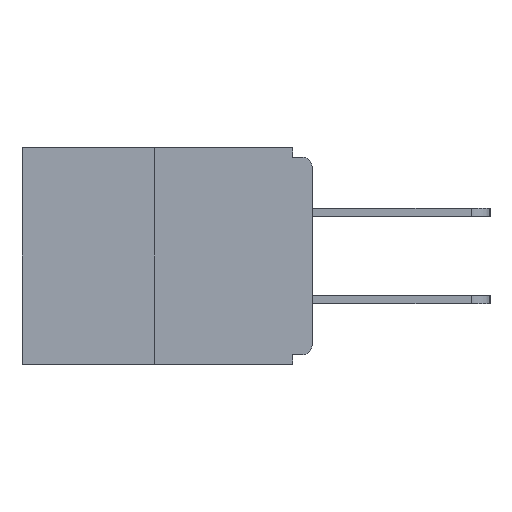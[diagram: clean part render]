
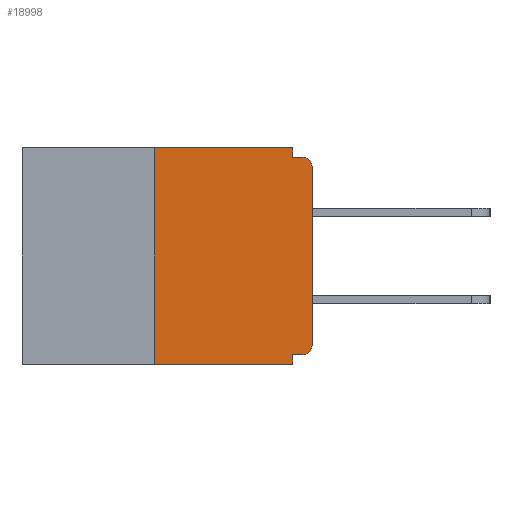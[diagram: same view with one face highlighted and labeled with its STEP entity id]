
A CAD part, left-side view. The second image highlights one B-rep face of the part: STEP entity #18998.
In plain terms, the highlighted planar face has unit normal (-1, 0, 0).
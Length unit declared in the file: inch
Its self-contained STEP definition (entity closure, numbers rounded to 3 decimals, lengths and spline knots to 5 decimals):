
#449 = DIRECTION ( 'NONE',  ( 0., 0., 1. ) ) ;
#732 = CARTESIAN_POINT ( 'NONE',  ( 0., 0.25, 0. ) ) ;
#2021 = CARTESIAN_POINT ( 'NONE',  ( 0., 0.25, -0.343 ) ) ;
#2976 = CARTESIAN_POINT ( 'NONE',  ( 0., 0., -0.328 ) ) ;
#3298 = LINE ( 'NONE', #7360, #22466 ) ;
#4478 = DIRECTION ( 'NONE',  ( 1., 0., 0. ) ) ;
#4510 = CARTESIAN_POINT ( 'NONE',  ( 0., 0.25, 0. ) ) ;
#4752 = VERTEX_POINT ( 'NONE', #18791 ) ;
#4906 = LINE ( 'NONE', #26805, #29667 ) ;
#4946 = EDGE_CURVE ( 'NONE', #25411, #9145, #12373, .T. ) ;
#5059 = EDGE_LOOP ( 'NONE', ( #11065, #24870, #18500, #27363, #10244, #5764, #27977, #21273, #30615, #14819 ) ) ;
#5166 = EDGE_CURVE ( 'NONE', #6661, #10984, #5220, .T. ) ;
#5220 = CIRCLE ( 'NONE', #25981, 0.015 ) ;
#5764 = ORIENTED_EDGE ( 'NONE', *, *, #5166, .T. ) ;
#6032 = FACE_OUTER_BOUND ( 'NONE', #5059, .T. ) ;
#6065 = DIRECTION ( 'NONE',  ( -1., 0., 0. ) ) ;
#6290 = CARTESIAN_POINT ( 'NONE',  ( 0., 0.031, 0. ) ) ;
#6461 = PLANE ( 'NONE',  #17625 ) ;
#6661 = VERTEX_POINT ( 'NONE', #27737 ) ;
#7360 = CARTESIAN_POINT ( 'NONE',  ( 0., 0., -0.015 ) ) ;
#7585 = VECTOR ( 'NONE', #449, 39.37008 ) ;
#9145 = VERTEX_POINT ( 'NONE', #24005 ) ;
#9698 = LINE ( 'NONE', #2976, #14955 ) ;
#10244 = ORIENTED_EDGE ( 'NONE', *, *, #13657, .F. ) ;
#10552 = CARTESIAN_POINT ( 'NONE',  ( 0., 0.46, -0.343 ) ) ;
#10764 = LINE ( 'NONE', #10552, #26503 ) ;
#10984 = VERTEX_POINT ( 'NONE', #27610 ) ;
#11065 = ORIENTED_EDGE ( 'NONE', *, *, #12440, .F. ) ;
#12373 = LINE ( 'NONE', #30499, #13145 ) ;
#12437 = DIRECTION ( 'NONE',  ( 0., -1., 0. ) ) ;
#12440 = EDGE_CURVE ( 'NONE', #20404, #25411, #4906, .T. ) ;
#12599 = CARTESIAN_POINT ( 'NONE',  ( 0., 0., -0.03 ) ) ;
#12611 = EDGE_CURVE ( 'NONE', #28470, #19201, #10764, .T. ) ;
#13145 = VECTOR ( 'NONE', #30386, 39.37008 ) ;
#13269 = CARTESIAN_POINT ( 'NONE',  ( 0., 0.031, -0.343 ) ) ;
#13657 = EDGE_CURVE ( 'NONE', #6661, #17230, #9698, .T. ) ;
#13726 = DIRECTION ( 'NONE',  ( 0., 0., -1. ) ) ;
#14003 = DIRECTION ( 'NONE',  ( 0., 0., -1. ) ) ;
#14268 = DIRECTION ( 'NONE',  ( 0., 0., 1. ) ) ;
#14388 = VECTOR ( 'NONE', #14268, 39.37008 ) ;
#14644 = CIRCLE ( 'NONE', #20902, 0.015 ) ;
#14819 = ORIENTED_EDGE ( 'NONE', *, *, #4946, .F. ) ;
#14955 = VECTOR ( 'NONE', #26798, 39.37008 ) ;
#15053 = DIRECTION ( 'NONE',  ( -1., 0., 0. ) ) ;
#15155 = CARTESIAN_POINT ( 'NONE',  ( 0., 0.015, -0.313 ) ) ;
#15611 = CARTESIAN_POINT ( 'NONE',  ( 0., 0.031, -0.328 ) ) ;
#16011 = DIRECTION ( 'NONE',  ( 0., 0., -1. ) ) ;
#16230 = LINE ( 'NONE', #19332, #7585 ) ;
#16352 = LINE ( 'NONE', #18699, #24613 ) ;
#17230 = VERTEX_POINT ( 'NONE', #15611 ) ;
#17379 = LINE ( 'NONE', #4510, #14388 ) ;
#17625 = AXIS2_PLACEMENT_3D ( 'NONE', #28490, #4478, #13726 ) ;
#17681 = EDGE_CURVE ( 'NONE', #10984, #21330, #16230, .T. ) ;
#18500 = ORIENTED_EDGE ( 'NONE', *, *, #12611, .T. ) ;
#18699 = CARTESIAN_POINT ( 'NONE',  ( 0., 0.031, -0.343 ) ) ;
#18791 = CARTESIAN_POINT ( 'NONE',  ( 0., 0.015, -0.015 ) ) ;
#18998 = ADVANCED_FACE ( 'NONE', ( #6032 ), #6461, .F. ) ;
#19201 = VERTEX_POINT ( 'NONE', #13269 ) ;
#19332 = CARTESIAN_POINT ( 'NONE',  ( 0., 0., 0. ) ) ;
#20404 = VERTEX_POINT ( 'NONE', #732 ) ;
#20902 = AXIS2_PLACEMENT_3D ( 'NONE', #30072, #6065, #16011 ) ;
#20904 = EDGE_CURVE ( 'NONE', #21330, #4752, #14644, .T. ) ;
#21273 = ORIENTED_EDGE ( 'NONE', *, *, #20904, .T. ) ;
#21330 = VERTEX_POINT ( 'NONE', #12599 ) ;
#22112 = EDGE_CURVE ( 'NONE', #9145, #4752, #3298, .T. ) ;
#22466 = VECTOR ( 'NONE', #24174, 39.37008 ) ;
#24005 = CARTESIAN_POINT ( 'NONE',  ( 0., 0.031, -0.015 ) ) ;
#24174 = DIRECTION ( 'NONE',  ( 0., -1., 0. ) ) ;
#24613 = VECTOR ( 'NONE', #14003, 39.37008 ) ;
#24870 = ORIENTED_EDGE ( 'NONE', *, *, #26268, .F. ) ;
#24959 = DIRECTION ( 'NONE',  ( 0., 0., -1. ) ) ;
#25411 = VERTEX_POINT ( 'NONE', #6290 ) ;
#25981 = AXIS2_PLACEMENT_3D ( 'NONE', #15155, #15053, #24959 ) ;
#26268 = EDGE_CURVE ( 'NONE', #28470, #20404, #17379, .T. ) ;
#26503 = VECTOR ( 'NONE', #27320, 39.37008 ) ;
#26798 = DIRECTION ( 'NONE',  ( 0., 1., 0. ) ) ;
#26805 = CARTESIAN_POINT ( 'NONE',  ( 0., 0.46, 0. ) ) ;
#27320 = DIRECTION ( 'NONE',  ( 0., -1., 0. ) ) ;
#27363 = ORIENTED_EDGE ( 'NONE', *, *, #30536, .F. ) ;
#27610 = CARTESIAN_POINT ( 'NONE',  ( 0., 0., -0.313 ) ) ;
#27737 = CARTESIAN_POINT ( 'NONE',  ( 0., 0.015, -0.328 ) ) ;
#27977 = ORIENTED_EDGE ( 'NONE', *, *, #17681, .T. ) ;
#28470 = VERTEX_POINT ( 'NONE', #2021 ) ;
#28490 = CARTESIAN_POINT ( 'NONE',  ( 0., 0.46, 0. ) ) ;
#29667 = VECTOR ( 'NONE', #12437, 39.37008 ) ;
#30072 = CARTESIAN_POINT ( 'NONE',  ( 0., 0.015, -0.03 ) ) ;
#30386 = DIRECTION ( 'NONE',  ( 0., 0., -1. ) ) ;
#30499 = CARTESIAN_POINT ( 'NONE',  ( 0., 0.031, 0. ) ) ;
#30536 = EDGE_CURVE ( 'NONE', #17230, #19201, #16352, .T. ) ;
#30615 = ORIENTED_EDGE ( 'NONE', *, *, #22112, .F. ) ;
